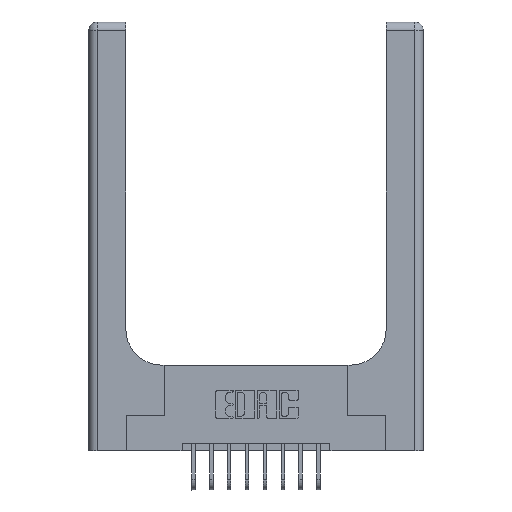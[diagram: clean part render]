
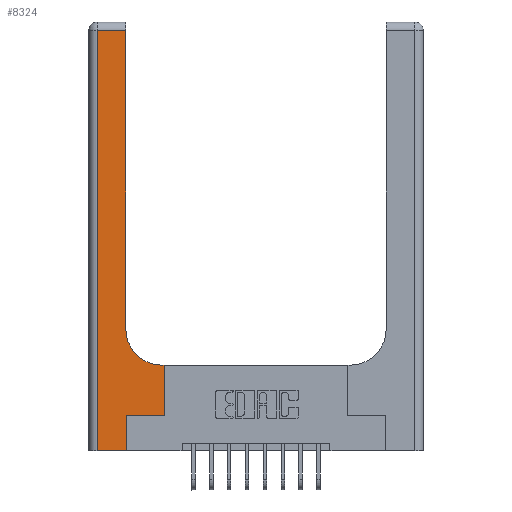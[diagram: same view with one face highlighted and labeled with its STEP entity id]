
A CAD part, top view. The second image highlights one B-rep face of the part: STEP entity #8324.
In plain terms, the highlighted planar face has unit normal (0, 0, 1).
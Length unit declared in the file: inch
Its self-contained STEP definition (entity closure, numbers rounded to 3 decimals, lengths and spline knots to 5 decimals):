
#325 = CARTESIAN_POINT ( 'NONE',  ( 0.06, 2.94, 0.37 ) ) ;
#1071 = EDGE_CURVE ( 'NONE', #1574, #12605, #9117, .T. ) ;
#1102 = EDGE_CURVE ( 'NONE', #1566, #1574, #1960, .T. ) ;
#1119 = EDGE_CURVE ( 'NONE', #8566, #1566, #14929, .T. ) ;
#1296 = VECTOR ( 'NONE', #10280, 39.37008 ) ;
#1481 = CARTESIAN_POINT ( 'NONE',  ( 0., 2.94, 0.37 ) ) ;
#1483 = CIRCLE ( 'NONE', #14801, 0.25 ) ;
#1501 = EDGE_LOOP ( 'NONE', ( #13149, #4082, #7795, #2601, #2421, #7884, #2386, #3360, #2164 ) ) ;
#1566 = VERTEX_POINT ( 'NONE', #7690 ) ;
#1574 = VERTEX_POINT ( 'NONE', #4497 ) ;
#1685 = CARTESIAN_POINT ( 'NONE',  ( 0.51, 0.6, 0.37 ) ) ;
#1778 = VECTOR ( 'NONE', #15209, 39.37008 ) ;
#1803 = CARTESIAN_POINT ( 'NONE',  ( 0.26, 2.94, 0.37 ) ) ;
#1960 = LINE ( 'NONE', #13547, #11890 ) ;
#2074 = DIRECTION ( 'NONE',  ( 0., 1., 0. ) ) ;
#2105 = VECTOR ( 'NONE', #4970, 39.37008 ) ;
#2164 = ORIENTED_EDGE ( 'NONE', *, *, #2956, .T. ) ;
#2386 = ORIENTED_EDGE ( 'NONE', *, *, #10805, .T. ) ;
#2421 = ORIENTED_EDGE ( 'NONE', *, *, #1071, .T. ) ;
#2601 = ORIENTED_EDGE ( 'NONE', *, *, #1102, .T. ) ;
#2922 = LINE ( 'NONE', #14891, #13637 ) ;
#2956 = EDGE_CURVE ( 'NONE', #4369, #13440, #1483, .T. ) ;
#3176 = CARTESIAN_POINT ( 'NONE',  ( 0.265, 0., 0.37 ) ) ;
#3360 = ORIENTED_EDGE ( 'NONE', *, *, #6078, .T. ) ;
#3739 = DIRECTION ( 'NONE',  ( 1., 0., 0. ) ) ;
#3800 = CARTESIAN_POINT ( 'NONE',  ( 0.265, 0.25, 0.37 ) ) ;
#3935 = EDGE_CURVE ( 'NONE', #13440, #8200, #6774, .T. ) ;
#4082 = ORIENTED_EDGE ( 'NONE', *, *, #5147, .T. ) ;
#4183 = DIRECTION ( 'NONE',  ( 0., 0., -1. ) ) ;
#4369 = VERTEX_POINT ( 'NONE', #1685 ) ;
#4461 = LINE ( 'NONE', #9161, #12683 ) ;
#4497 = CARTESIAN_POINT ( 'NONE',  ( 0.265, 0., 0.37 ) ) ;
#4970 = DIRECTION ( 'NONE',  ( 1., 0., 0. ) ) ;
#5147 = EDGE_CURVE ( 'NONE', #8200, #8566, #8492, .T. ) ;
#5410 = CARTESIAN_POINT ( 'NONE',  ( 0., 3., 0.37 ) ) ;
#6078 = EDGE_CURVE ( 'NONE', #7498, #4369, #4461, .T. ) ;
#6231 = EDGE_CURVE ( 'NONE', #12605, #6522, #6286, .T. ) ;
#6286 = LINE ( 'NONE', #11083, #2105 ) ;
#6522 = VERTEX_POINT ( 'NONE', #10528 ) ;
#6774 = LINE ( 'NONE', #8152, #1778 ) ;
#7498 = VERTEX_POINT ( 'NONE', #11477 ) ;
#7690 = CARTESIAN_POINT ( 'NONE',  ( 0.06, 0., 0.37 ) ) ;
#7783 = CARTESIAN_POINT ( 'NONE',  ( 0.26, 0.85, 0.37 ) ) ;
#7795 = ORIENTED_EDGE ( 'NONE', *, *, #1119, .T. ) ;
#7884 = ORIENTED_EDGE ( 'NONE', *, *, #6231, .T. ) ;
#7956 = CARTESIAN_POINT ( 'NONE',  ( 0.06, 3., 0.37 ) ) ;
#8008 = DIRECTION ( 'NONE',  ( -1., 0., 0. ) ) ;
#8152 = CARTESIAN_POINT ( 'NONE',  ( 0.26, 3., 0.37 ) ) ;
#8200 = VERTEX_POINT ( 'NONE', #1803 ) ;
#8227 = VECTOR ( 'NONE', #11123, 39.37008 ) ;
#8309 = CARTESIAN_POINT ( 'NONE',  ( 0.51, 0.85, 0.37 ) ) ;
#8324 = ADVANCED_FACE ( 'NONE', ( #14767 ), #10278, .F. ) ;
#8492 = LINE ( 'NONE', #1481, #8227 ) ;
#8566 = VERTEX_POINT ( 'NONE', #325 ) ;
#8759 = AXIS2_PLACEMENT_3D ( 'NONE', #5410, #4183, #12540 ) ;
#9117 = LINE ( 'NONE', #3176, #1296 ) ;
#9161 = CARTESIAN_POINT ( 'NONE',  ( 0.26, 0.6, 0.37 ) ) ;
#10278 = PLANE ( 'NONE',  #8759 ) ;
#10280 = DIRECTION ( 'NONE',  ( 0., 1., 0. ) ) ;
#10394 = VECTOR ( 'NONE', #11213, 39.37008 ) ;
#10528 = CARTESIAN_POINT ( 'NONE',  ( 0.528, 0.25, 0.37 ) ) ;
#10805 = EDGE_CURVE ( 'NONE', #6522, #7498, #2922, .T. ) ;
#11083 = CARTESIAN_POINT ( 'NONE',  ( 0.265, 0.25, 0.37 ) ) ;
#11123 = DIRECTION ( 'NONE',  ( -1., 0., 0. ) ) ;
#11213 = DIRECTION ( 'NONE',  ( 0., -1., 0. ) ) ;
#11477 = CARTESIAN_POINT ( 'NONE',  ( 0.528, 0.6, 0.37 ) ) ;
#11890 = VECTOR ( 'NONE', #12463, 39.37008 ) ;
#12463 = DIRECTION ( 'NONE',  ( 1., 0., 0. ) ) ;
#12540 = DIRECTION ( 'NONE',  ( -1., 0., 0. ) ) ;
#12605 = VERTEX_POINT ( 'NONE', #3800 ) ;
#12683 = VECTOR ( 'NONE', #8008, 39.37008 ) ;
#13026 = DIRECTION ( 'NONE',  ( 0., 0., -1. ) ) ;
#13149 = ORIENTED_EDGE ( 'NONE', *, *, #3935, .T. ) ;
#13440 = VERTEX_POINT ( 'NONE', #7783 ) ;
#13547 = CARTESIAN_POINT ( 'NONE',  ( 0., 0., 0.37 ) ) ;
#13637 = VECTOR ( 'NONE', #2074, 39.37008 ) ;
#14767 = FACE_OUTER_BOUND ( 'NONE', #1501, .T. ) ;
#14801 = AXIS2_PLACEMENT_3D ( 'NONE', #8309, #13026, #3739 ) ;
#14891 = CARTESIAN_POINT ( 'NONE',  ( 0.528, 0.25, 0.37 ) ) ;
#14929 = LINE ( 'NONE', #7956, #10394 ) ;
#15209 = DIRECTION ( 'NONE',  ( 0., 1., 0. ) ) ;
